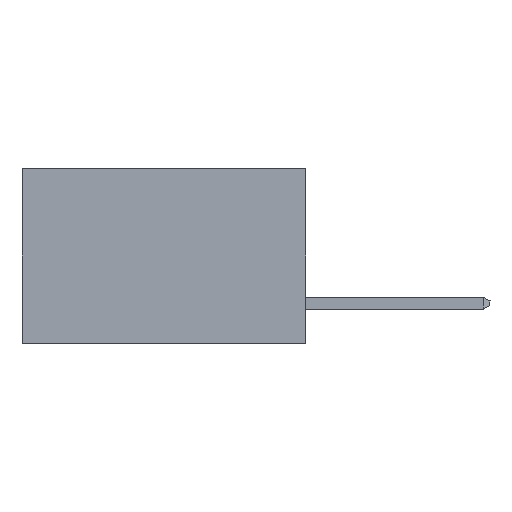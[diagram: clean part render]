
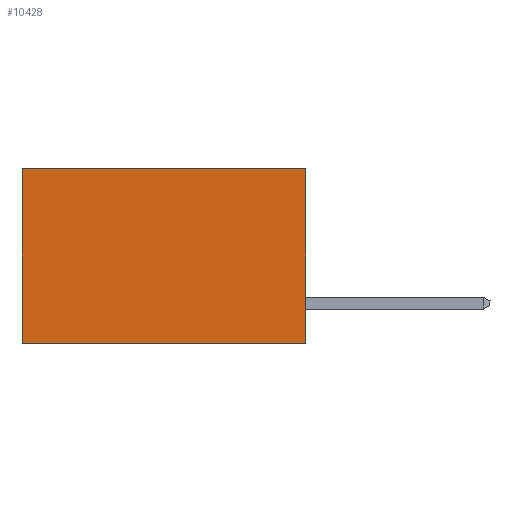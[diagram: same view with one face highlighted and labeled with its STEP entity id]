
A CAD part, left-side view. The second image highlights one B-rep face of the part: STEP entity #10428.
In plain terms, the highlighted planar face has unit normal (-1, 0, 0).
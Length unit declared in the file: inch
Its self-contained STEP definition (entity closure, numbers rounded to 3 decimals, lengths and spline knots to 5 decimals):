
#547 = VECTOR ( 'NONE', #4721, 39.37008 ) ;
#585 = VECTOR ( 'NONE', #19303, 39.37008 ) ;
#1213 = VERTEX_POINT ( 'NONE', #28509 ) ;
#1329 = LINE ( 'NONE', #2271, #547 ) ;
#1667 = EDGE_CURVE ( 'NONE', #1213, #14498, #1329, .T. ) ;
#1684 = PLANE ( 'NONE',  #6903 ) ;
#2271 = CARTESIAN_POINT ( 'NONE',  ( 0.298, 0., -0.37 ) ) ;
#3003 = CARTESIAN_POINT ( 'NONE',  ( 0.298, 0.6, 0. ) ) ;
#3308 = CARTESIAN_POINT ( 'NONE',  ( 0.298, 0.6, 0. ) ) ;
#3783 = ORIENTED_EDGE ( 'NONE', *, *, #6597, .F. ) ;
#4721 = DIRECTION ( 'NONE',  ( 0., 1., 0. ) ) ;
#4730 = EDGE_CURVE ( 'NONE', #31216, #14498, #31586, .T. ) ;
#5649 = DIRECTION ( 'NONE',  ( 0., 0., -1. ) ) ;
#6129 = LINE ( 'NONE', #16665, #24773 ) ;
#6597 = EDGE_CURVE ( 'NONE', #22104, #1213, #6129, .T. ) ;
#6903 = AXIS2_PLACEMENT_3D ( 'NONE', #20841, #23646, #23537 ) ;
#8904 = FACE_OUTER_BOUND ( 'NONE', #20182, .T. ) ;
#10428 = ADVANCED_FACE ( 'NONE', ( #8904 ), #1684, .F. ) ;
#10573 = CARTESIAN_POINT ( 'NONE',  ( 0.298, 0.6, -0.37 ) ) ;
#14498 = VERTEX_POINT ( 'NONE', #10573 ) ;
#14824 = CARTESIAN_POINT ( 'NONE',  ( 0.298, 0., 0. ) ) ;
#16665 = CARTESIAN_POINT ( 'NONE',  ( 0.298, 0., 0. ) ) ;
#17071 = ORIENTED_EDGE ( 'NONE', *, *, #26483, .T. ) ;
#19303 = DIRECTION ( 'NONE',  ( 0., 1., 0. ) ) ;
#19537 = DIRECTION ( 'NONE',  ( 0., 0., -1. ) ) ;
#20182 = EDGE_LOOP ( 'NONE', ( #28000, #28640, #3783, #17071 ) ) ;
#20841 = CARTESIAN_POINT ( 'NONE',  ( 0.298, 0., 0. ) ) ;
#22104 = VERTEX_POINT ( 'NONE', #23569 ) ;
#23537 = DIRECTION ( 'NONE',  ( 0., 0., -1. ) ) ;
#23569 = CARTESIAN_POINT ( 'NONE',  ( 0.298, 0., 0. ) ) ;
#23646 = DIRECTION ( 'NONE',  ( 1., 0., 0. ) ) ;
#24337 = VECTOR ( 'NONE', #5649, 39.37008 ) ;
#24773 = VECTOR ( 'NONE', #19537, 39.37008 ) ;
#26170 = LINE ( 'NONE', #14824, #585 ) ;
#26483 = EDGE_CURVE ( 'NONE', #22104, #31216, #26170, .T. ) ;
#28000 = ORIENTED_EDGE ( 'NONE', *, *, #4730, .T. ) ;
#28509 = CARTESIAN_POINT ( 'NONE',  ( 0.298, 0., -0.37 ) ) ;
#28640 = ORIENTED_EDGE ( 'NONE', *, *, #1667, .F. ) ;
#31216 = VERTEX_POINT ( 'NONE', #3308 ) ;
#31586 = LINE ( 'NONE', #3003, #24337 ) ;
